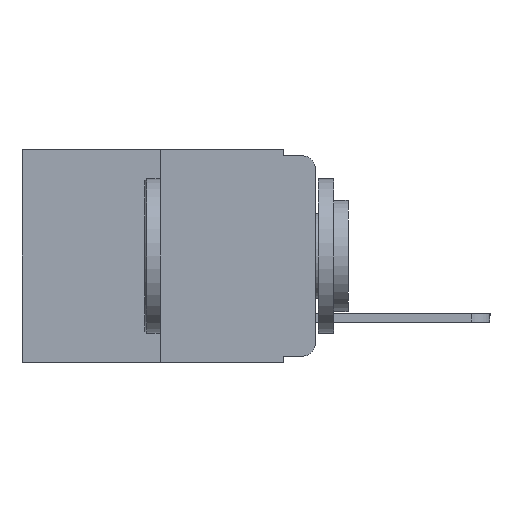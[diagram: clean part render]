
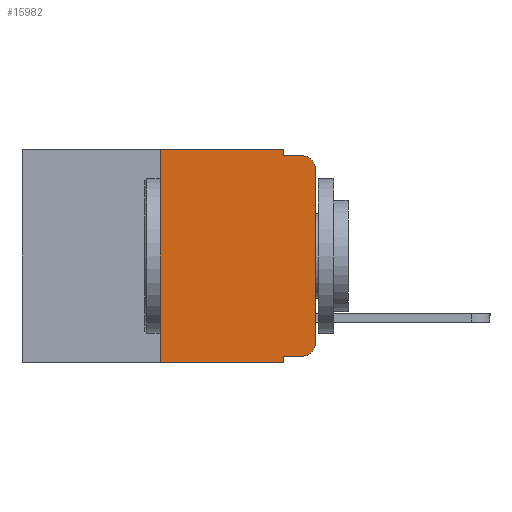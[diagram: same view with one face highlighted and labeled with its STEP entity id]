
A CAD part, left-side view. The second image highlights one B-rep face of the part: STEP entity #15982.
In plain terms, the highlighted planar face has unit normal (-1, 0, 0).
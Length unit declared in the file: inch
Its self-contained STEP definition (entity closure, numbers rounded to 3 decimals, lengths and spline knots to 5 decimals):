
#322 = EDGE_CURVE ( 'NONE', #3963, #6676, #9869, .T. ) ;
#363 = EDGE_CURVE ( 'NONE', #10760, #3963, #16898, .T. ) ;
#421 = DIRECTION ( 'NONE',  ( 0., 0., -1. ) ) ;
#505 = DIRECTION ( 'NONE',  ( 0., -1., 0. ) ) ;
#856 = ORIENTED_EDGE ( 'NONE', *, *, #2501, .F. ) ;
#1101 = VERTEX_POINT ( 'NONE', #1598 ) ;
#1261 = EDGE_CURVE ( 'NONE', #18349, #3497, #6284, .T. ) ;
#1508 = CARTESIAN_POINT ( 'NONE',  ( 0., 0.473, 0. ) ) ;
#1569 = EDGE_CURVE ( 'NONE', #10760, #1101, #15367, .T. ) ;
#1598 = CARTESIAN_POINT ( 'NONE',  ( 0., 0.051, -0.343 ) ) ;
#1656 = VECTOR ( 'NONE', #19793, 39.37008 ) ;
#1721 = EDGE_CURVE ( 'NONE', #16080, #18349, #7570, .T. ) ;
#1768 = DIRECTION ( 'NONE',  ( -1., 0., 0. ) ) ;
#2090 = ORIENTED_EDGE ( 'NONE', *, *, #1721, .F. ) ;
#2501 = EDGE_CURVE ( 'NONE', #3497, #18401, #14296, .T. ) ;
#3052 = CARTESIAN_POINT ( 'NONE',  ( 0., 0.051, 0. ) ) ;
#3098 = VECTOR ( 'NONE', #13010, 39.37008 ) ;
#3294 = EDGE_CURVE ( 'NONE', #18401, #20031, #8205, .T. ) ;
#3360 = CARTESIAN_POINT ( 'NONE',  ( 0., 0.051, -0.333 ) ) ;
#3468 = EDGE_CURVE ( 'NONE', #14089, #20031, #20641, .T. ) ;
#3472 = EDGE_CURVE ( 'NONE', #6676, #14089, #12241, .T. ) ;
#3497 = VERTEX_POINT ( 'NONE', #3052 ) ;
#3963 = VERTEX_POINT ( 'NONE', #21356 ) ;
#4103 = CARTESIAN_POINT ( 'NONE',  ( 0., 0., 0. ) ) ;
#6161 = CARTESIAN_POINT ( 'NONE',  ( 0., 0.02, -0.313 ) ) ;
#6284 = LINE ( 'NONE', #1508, #1656 ) ;
#6676 = VERTEX_POINT ( 'NONE', #21400 ) ;
#6957 = CARTESIAN_POINT ( 'NONE',  ( 0., 0.051, -0.333 ) ) ;
#7570 = LINE ( 'NONE', #16556, #3098 ) ;
#7584 = CARTESIAN_POINT ( 'NONE',  ( 0., 0.25, 0. ) ) ;
#7627 = VECTOR ( 'NONE', #505, 39.37008 ) ;
#7720 = ORIENTED_EDGE ( 'NONE', *, *, #363, .T. ) ;
#8183 = CARTESIAN_POINT ( 'NONE',  ( 0., 0.473, 0. ) ) ;
#8205 = LINE ( 'NONE', #16618, #12008 ) ;
#8257 = PLANE ( 'NONE',  #16107 ) ;
#8951 = ORIENTED_EDGE ( 'NONE', *, *, #3468, .T. ) ;
#9663 = FACE_OUTER_BOUND ( 'NONE', #20427, .T. ) ;
#9869 = CIRCLE ( 'NONE', #15268, 0.02 ) ;
#9874 = DIRECTION ( 'NONE',  ( 0., 0., -1. ) ) ;
#10760 = VERTEX_POINT ( 'NONE', #6957 ) ;
#10991 = ORIENTED_EDGE ( 'NONE', *, *, #21351, .T. ) ;
#11103 = VECTOR ( 'NONE', #11134, 39.37008 ) ;
#11134 = DIRECTION ( 'NONE',  ( 0., 0., -1. ) ) ;
#12008 = VECTOR ( 'NONE', #16445, 39.37008 ) ;
#12022 = ORIENTED_EDGE ( 'NONE', *, *, #322, .T. ) ;
#12147 = CARTESIAN_POINT ( 'NONE',  ( 0., 0.051, 0. ) ) ;
#12241 = LINE ( 'NONE', #4103, #20142 ) ;
#12646 = VECTOR ( 'NONE', #21453, 39.37008 ) ;
#13010 = DIRECTION ( 'NONE',  ( 0., 0., 1. ) ) ;
#13255 = ORIENTED_EDGE ( 'NONE', *, *, #3294, .F. ) ;
#13316 = CARTESIAN_POINT ( 'NONE',  ( 0., 0., -0.03 ) ) ;
#13324 = CARTESIAN_POINT ( 'NONE',  ( 0., 0.25, -0.343 ) ) ;
#13432 = DIRECTION ( 'NONE',  ( 0., 0., 1. ) ) ;
#13792 = VECTOR ( 'NONE', #21349, 39.37008 ) ;
#14089 = VERTEX_POINT ( 'NONE', #13316 ) ;
#14177 = DIRECTION ( 'NONE',  ( 0., 0., -1. ) ) ;
#14296 = LINE ( 'NONE', #12147, #13792 ) ;
#14436 = DIRECTION ( 'NONE',  ( -1., 0., 0. ) ) ;
#14509 = CARTESIAN_POINT ( 'NONE',  ( 0., 0.02, -0.03 ) ) ;
#15268 = AXIS2_PLACEMENT_3D ( 'NONE', #6161, #1768, #421 ) ;
#15367 = LINE ( 'NONE', #16034, #11103 ) ;
#15719 = CARTESIAN_POINT ( 'NONE',  ( 0., 0.02, -0.01 ) ) ;
#15743 = ORIENTED_EDGE ( 'NONE', *, *, #1569, .F. ) ;
#15982 = ADVANCED_FACE ( 'NONE', ( #9663 ), #8257, .F. ) ;
#16034 = CARTESIAN_POINT ( 'NONE',  ( 0., 0.051, 0. ) ) ;
#16080 = VERTEX_POINT ( 'NONE', #13324 ) ;
#16107 = AXIS2_PLACEMENT_3D ( 'NONE', #8183, #19407, #9874 ) ;
#16445 = DIRECTION ( 'NONE',  ( 0., -1., 0. ) ) ;
#16556 = CARTESIAN_POINT ( 'NONE',  ( 0., 0.25, 0. ) ) ;
#16618 = CARTESIAN_POINT ( 'NONE',  ( 0., 0.051, -0.01 ) ) ;
#16898 = LINE ( 'NONE', #3360, #12646 ) ;
#16991 = ORIENTED_EDGE ( 'NONE', *, *, #3472, .T. ) ;
#18349 = VERTEX_POINT ( 'NONE', #7584 ) ;
#18401 = VERTEX_POINT ( 'NONE', #20368 ) ;
#18469 = ORIENTED_EDGE ( 'NONE', *, *, #1261, .F. ) ;
#19407 = DIRECTION ( 'NONE',  ( 1., 0., 0. ) ) ;
#19793 = DIRECTION ( 'NONE',  ( 0., -1., 0. ) ) ;
#20031 = VERTEX_POINT ( 'NONE', #15719 ) ;
#20142 = VECTOR ( 'NONE', #13432, 39.37008 ) ;
#20274 = CARTESIAN_POINT ( 'NONE',  ( 0., 0.473, -0.343 ) ) ;
#20312 = LINE ( 'NONE', #20274, #7627 ) ;
#20368 = CARTESIAN_POINT ( 'NONE',  ( 0., 0.051, -0.01 ) ) ;
#20427 = EDGE_LOOP ( 'NONE', ( #16991, #8951, #13255, #856, #18469, #2090, #10991, #15743, #7720, #12022 ) ) ;
#20641 = CIRCLE ( 'NONE', #21010, 0.02 ) ;
#21010 = AXIS2_PLACEMENT_3D ( 'NONE', #14509, #14436, #14177 ) ;
#21349 = DIRECTION ( 'NONE',  ( 0., 0., -1. ) ) ;
#21351 = EDGE_CURVE ( 'NONE', #16080, #1101, #20312, .T. ) ;
#21356 = CARTESIAN_POINT ( 'NONE',  ( 0., 0.02, -0.333 ) ) ;
#21400 = CARTESIAN_POINT ( 'NONE',  ( 0., 0., -0.313 ) ) ;
#21453 = DIRECTION ( 'NONE',  ( 0., -1., 0. ) ) ;
